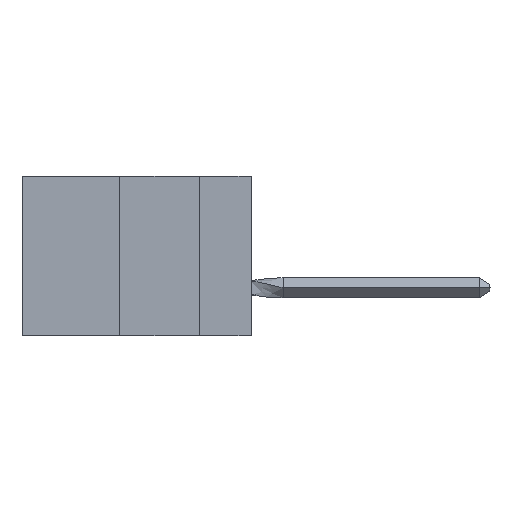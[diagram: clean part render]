
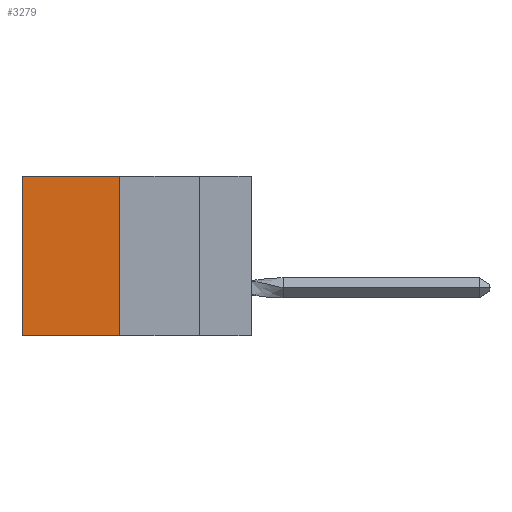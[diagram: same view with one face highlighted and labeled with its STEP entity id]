
A CAD part, left-side view. The second image highlights one B-rep face of the part: STEP entity #3279.
In plain terms, the highlighted planar face has unit normal (-1, 0, 0).
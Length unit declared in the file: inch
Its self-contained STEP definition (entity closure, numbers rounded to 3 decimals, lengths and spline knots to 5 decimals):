
#73 = VERTEX_POINT ( 'NONE', #6757 ) ;
#169 = ORIENTED_EDGE ( 'NONE', *, *, #21049, .T. ) ;
#242 = EDGE_CURVE ( 'NONE', #73, #14214, #14766, .T. ) ;
#1629 = VECTOR ( 'NONE', #9472, 39.37008 ) ;
#1820 = DIRECTION ( 'NONE',  ( 1., 0., 0. ) ) ;
#3279 = ADVANCED_FACE ( 'NONE', ( #8749 ), #8858, .F. ) ;
#3342 = CARTESIAN_POINT ( 'NONE',  ( 0.305, 0.413, -0.5 ) ) ;
#3827 = LINE ( 'NONE', #11078, #1629 ) ;
#3879 = DIRECTION ( 'NONE',  ( 0., 0., -1. ) ) ;
#4103 = EDGE_LOOP ( 'NONE', ( #14486, #17007, #11224, #169 ) ) ;
#4265 = EDGE_CURVE ( 'NONE', #13722, #73, #7937, .T. ) ;
#4576 = VERTEX_POINT ( 'NONE', #9044 ) ;
#5386 = CARTESIAN_POINT ( 'NONE',  ( 0.305, 0.413, -0.5 ) ) ;
#6757 = CARTESIAN_POINT ( 'NONE',  ( 0.305, 0.413, -0.5 ) ) ;
#7020 = EDGE_CURVE ( 'NONE', #4576, #14214, #10750, .T. ) ;
#7937 = LINE ( 'NONE', #3342, #17512 ) ;
#8749 = FACE_OUTER_BOUND ( 'NONE', #4103, .T. ) ;
#8858 = PLANE ( 'NONE',  #11213 ) ;
#9044 = CARTESIAN_POINT ( 'NONE',  ( 0.305, 0.72, 0. ) ) ;
#9472 = DIRECTION ( 'NONE',  ( 0., 1., 0. ) ) ;
#9477 = CARTESIAN_POINT ( 'NONE',  ( 0.305, 0.72, -0.5 ) ) ;
#9567 = VECTOR ( 'NONE', #19410, 39.37008 ) ;
#10450 = DIRECTION ( 'NONE',  ( 0., 0., -1. ) ) ;
#10750 = LINE ( 'NONE', #9477, #21493 ) ;
#11078 = CARTESIAN_POINT ( 'NONE',  ( 0.305, 0.413, 0. ) ) ;
#11213 = AXIS2_PLACEMENT_3D ( 'NONE', #21079, #1820, #12272 ) ;
#11224 = ORIENTED_EDGE ( 'NONE', *, *, #4265, .F. ) ;
#12272 = DIRECTION ( 'NONE',  ( 0., 0., -1. ) ) ;
#13722 = VERTEX_POINT ( 'NONE', #21212 ) ;
#14214 = VERTEX_POINT ( 'NONE', #19028 ) ;
#14486 = ORIENTED_EDGE ( 'NONE', *, *, #7020, .T. ) ;
#14766 = LINE ( 'NONE', #5386, #9567 ) ;
#17007 = ORIENTED_EDGE ( 'NONE', *, *, #242, .F. ) ;
#17512 = VECTOR ( 'NONE', #10450, 39.37008 ) ;
#19028 = CARTESIAN_POINT ( 'NONE',  ( 0.305, 0.72, -0.5 ) ) ;
#19410 = DIRECTION ( 'NONE',  ( 0., 1., 0. ) ) ;
#21049 = EDGE_CURVE ( 'NONE', #13722, #4576, #3827, .T. ) ;
#21079 = CARTESIAN_POINT ( 'NONE',  ( 0.305, 0.413, -0.5 ) ) ;
#21212 = CARTESIAN_POINT ( 'NONE',  ( 0.305, 0.413, 0. ) ) ;
#21493 = VECTOR ( 'NONE', #3879, 39.37008 ) ;
